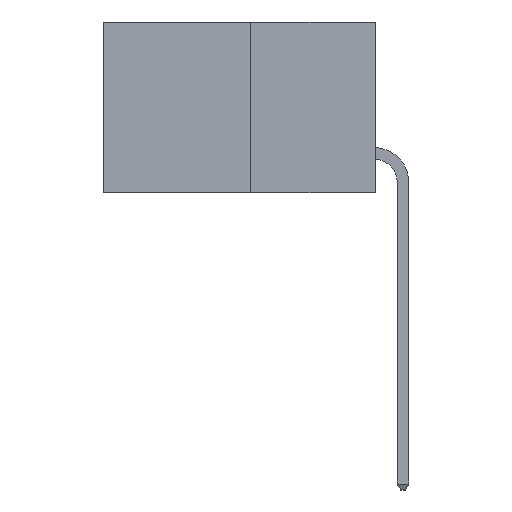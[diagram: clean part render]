
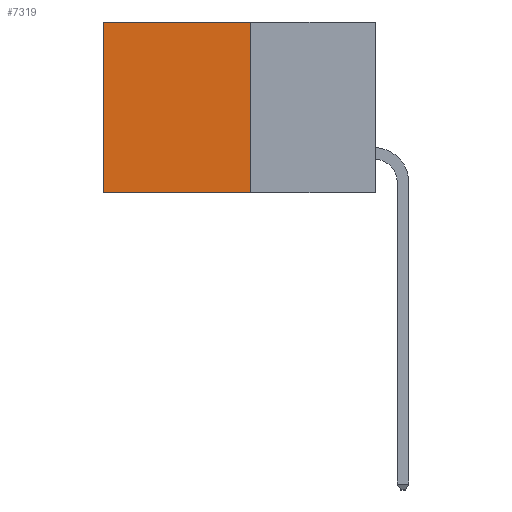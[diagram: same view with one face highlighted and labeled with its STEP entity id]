
A CAD part, left-side view. The second image highlights one B-rep face of the part: STEP entity #7319.
In plain terms, the highlighted planar face has unit normal (-1, 0, 0).
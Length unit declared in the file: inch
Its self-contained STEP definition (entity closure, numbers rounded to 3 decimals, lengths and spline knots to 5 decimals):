
#303 = CARTESIAN_POINT ( 'NONE',  ( 0.277, 0.27, -0.37 ) ) ;
#419 = CARTESIAN_POINT ( 'NONE',  ( 0.277, 0.59, 0. ) ) ;
#742 = AXIS2_PLACEMENT_3D ( 'NONE', #303, #2232, #8914 ) ;
#1027 = VECTOR ( 'NONE', #6073, 39.37008 ) ;
#1180 = DIRECTION ( 'NONE',  ( 0., 0., -1. ) ) ;
#1236 = CARTESIAN_POINT ( 'NONE',  ( 0.277, 0.27, -0.37 ) ) ;
#1282 = PLANE ( 'NONE',  #742 ) ;
#1758 = EDGE_CURVE ( 'NONE', #12110, #5549, #5898, .T. ) ;
#1782 = ORIENTED_EDGE ( 'NONE', *, *, #11207, .T. ) ;
#2232 = DIRECTION ( 'NONE',  ( 1., 0., 0. ) ) ;
#2286 = LINE ( 'NONE', #1236, #6795 ) ;
#3273 = LINE ( 'NONE', #10752, #1027 ) ;
#3783 = ORIENTED_EDGE ( 'NONE', *, *, #6883, .F. ) ;
#4062 = CARTESIAN_POINT ( 'NONE',  ( 0.277, 0.27, 0. ) ) ;
#4240 = FACE_OUTER_BOUND ( 'NONE', #6503, .T. ) ;
#4394 = ORIENTED_EDGE ( 'NONE', *, *, #1758, .F. ) ;
#4513 = CARTESIAN_POINT ( 'NONE',  ( 0.277, 0.27, -0.37 ) ) ;
#5549 = VERTEX_POINT ( 'NONE', #10810 ) ;
#5898 = LINE ( 'NONE', #10477, #8411 ) ;
#5917 = ORIENTED_EDGE ( 'NONE', *, *, #9133, .T. ) ;
#6073 = DIRECTION ( 'NONE',  ( 0., 0., -1. ) ) ;
#6354 = CARTESIAN_POINT ( 'NONE',  ( 0.277, 0.27, 0. ) ) ;
#6503 = EDGE_LOOP ( 'NONE', ( #5917, #4394, #3783, #1782 ) ) ;
#6795 = VECTOR ( 'NONE', #1180, 39.37008 ) ;
#6883 = EDGE_CURVE ( 'NONE', #10224, #12110, #2286, .T. ) ;
#7319 = ADVANCED_FACE ( 'NONE', ( #4240 ), #1282, .F. ) ;
#7612 = LINE ( 'NONE', #4062, #9796 ) ;
#7904 = DIRECTION ( 'NONE',  ( 0., 1., 0. ) ) ;
#8411 = VECTOR ( 'NONE', #11352, 39.37008 ) ;
#8914 = DIRECTION ( 'NONE',  ( 0., 0., -1. ) ) ;
#9133 = EDGE_CURVE ( 'NONE', #10653, #5549, #3273, .T. ) ;
#9796 = VECTOR ( 'NONE', #7904, 39.37008 ) ;
#10224 = VERTEX_POINT ( 'NONE', #6354 ) ;
#10477 = CARTESIAN_POINT ( 'NONE',  ( 0.277, 0.27, -0.37 ) ) ;
#10653 = VERTEX_POINT ( 'NONE', #419 ) ;
#10752 = CARTESIAN_POINT ( 'NONE',  ( 0.277, 0.59, -0.37 ) ) ;
#10810 = CARTESIAN_POINT ( 'NONE',  ( 0.277, 0.59, -0.37 ) ) ;
#11207 = EDGE_CURVE ( 'NONE', #10224, #10653, #7612, .T. ) ;
#11352 = DIRECTION ( 'NONE',  ( 0., 1., 0. ) ) ;
#12110 = VERTEX_POINT ( 'NONE', #4513 ) ;
